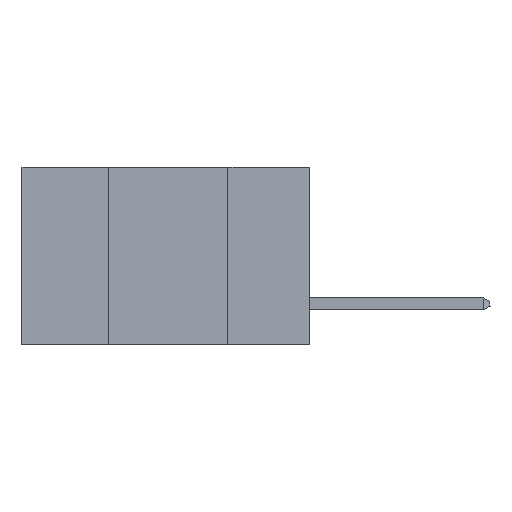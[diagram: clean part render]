
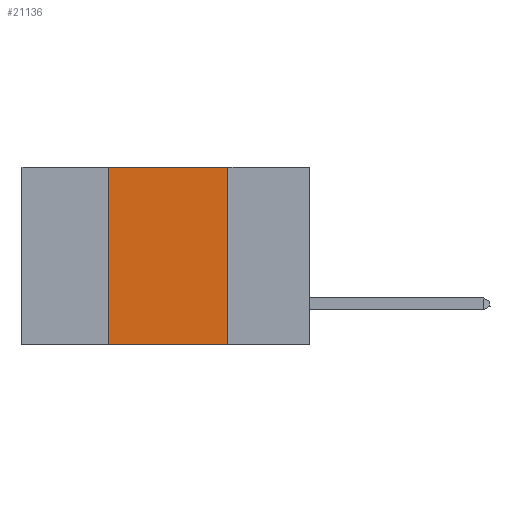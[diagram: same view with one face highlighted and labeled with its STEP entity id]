
A CAD part, left-side view. The second image highlights one B-rep face of the part: STEP entity #21136.
In plain terms, the highlighted planar face has unit normal (-1, 0, 0).
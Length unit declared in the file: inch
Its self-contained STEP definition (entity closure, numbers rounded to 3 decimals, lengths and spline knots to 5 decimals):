
#575 = CARTESIAN_POINT ( 'NONE',  ( 0., 0.6, -0.37 ) ) ;
#649 = CARTESIAN_POINT ( 'NONE',  ( 0., 0.17, -0.37 ) ) ;
#803 = DIRECTION ( 'NONE',  ( 0., -1., 0. ) ) ;
#2221 = CARTESIAN_POINT ( 'NONE',  ( 0., 0.17, 0. ) ) ;
#3432 = VERTEX_POINT ( 'NONE', #649 ) ;
#3765 = CARTESIAN_POINT ( 'NONE',  ( 0., 0.17, 0. ) ) ;
#4028 = VECTOR ( 'NONE', #803, 39.37008 ) ;
#5371 = CARTESIAN_POINT ( 'NONE',  ( 0., 0.42, 0. ) ) ;
#5445 = LINE ( 'NONE', #12422, #11029 ) ;
#6882 = DIRECTION ( 'NONE',  ( 0., -1., 0. ) ) ;
#8401 = LINE ( 'NONE', #575, #4028 ) ;
#9061 = FACE_OUTER_BOUND ( 'NONE', #16464, .T. ) ;
#9686 = CARTESIAN_POINT ( 'NONE',  ( 0., 0.6, 0. ) ) ;
#11029 = VECTOR ( 'NONE', #6882, 39.37008 ) ;
#11100 = CARTESIAN_POINT ( 'NONE',  ( 0., 0.42, -0.37 ) ) ;
#11408 = EDGE_CURVE ( 'NONE', #18230, #13358, #25760, .T. ) ;
#11590 = VECTOR ( 'NONE', #22048, 39.37008 ) ;
#11892 = ORIENTED_EDGE ( 'NONE', *, *, #28178, .F. ) ;
#12422 = CARTESIAN_POINT ( 'NONE',  ( 0., 0.6, 0. ) ) ;
#13358 = VERTEX_POINT ( 'NONE', #5371 ) ;
#14988 = EDGE_CURVE ( 'NONE', #27682, #3432, #25149, .T. ) ;
#16464 = EDGE_LOOP ( 'NONE', ( #16597, #11892, #29006, #21234 ) ) ;
#16597 = ORIENTED_EDGE ( 'NONE', *, *, #14988, .F. ) ;
#17234 = DIRECTION ( 'NONE',  ( 1., 0., 0. ) ) ;
#18230 = VERTEX_POINT ( 'NONE', #11100 ) ;
#19474 = DIRECTION ( 'NONE',  ( 0., 0., -1. ) ) ;
#20616 = DIRECTION ( 'NONE',  ( 0., 0., 1. ) ) ;
#21136 = ADVANCED_FACE ( 'NONE', ( #9061 ), #22174, .F. ) ;
#21234 = ORIENTED_EDGE ( 'NONE', *, *, #26655, .T. ) ;
#22048 = DIRECTION ( 'NONE',  ( 0., 0., -1. ) ) ;
#22174 = PLANE ( 'NONE',  #27688 ) ;
#25149 = LINE ( 'NONE', #3765, #11590 ) ;
#25298 = CARTESIAN_POINT ( 'NONE',  ( 0., 0.42, 0. ) ) ;
#25760 = LINE ( 'NONE', #25298, #32929 ) ;
#26655 = EDGE_CURVE ( 'NONE', #18230, #3432, #8401, .T. ) ;
#27682 = VERTEX_POINT ( 'NONE', #2221 ) ;
#27688 = AXIS2_PLACEMENT_3D ( 'NONE', #9686, #17234, #19474 ) ;
#28178 = EDGE_CURVE ( 'NONE', #13358, #27682, #5445, .T. ) ;
#29006 = ORIENTED_EDGE ( 'NONE', *, *, #11408, .F. ) ;
#32929 = VECTOR ( 'NONE', #20616, 39.37008 ) ;
